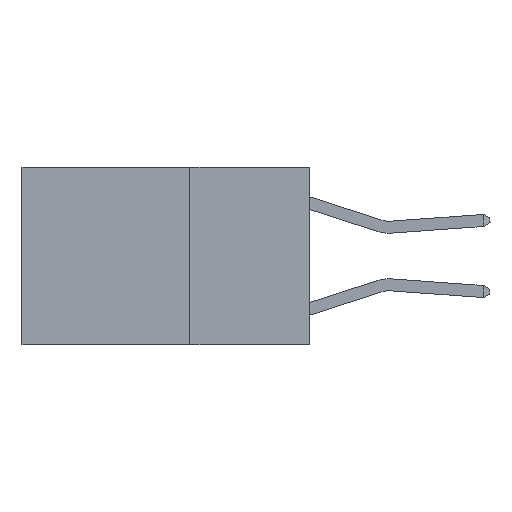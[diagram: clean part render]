
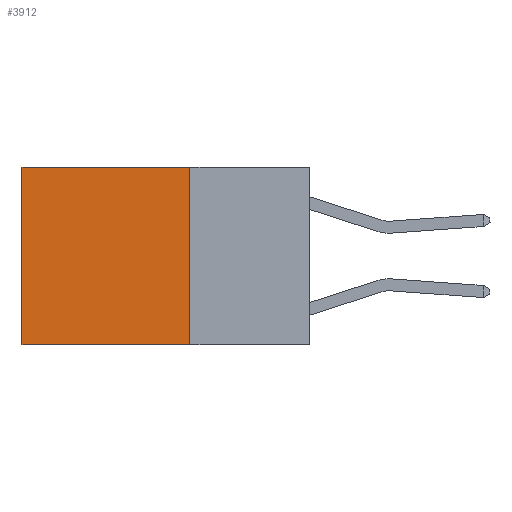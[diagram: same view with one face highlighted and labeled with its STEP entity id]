
A CAD part, left-side view. The second image highlights one B-rep face of the part: STEP entity #3912.
In plain terms, the highlighted planar face has unit normal (-1, 0, 0).
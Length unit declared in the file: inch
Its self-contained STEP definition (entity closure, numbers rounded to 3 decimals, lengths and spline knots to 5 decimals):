
#77 = EDGE_LOOP ( 'NONE', ( #11170, #1168, #11454, #1470 ) ) ;
#141 = VECTOR ( 'NONE', #8031, 39.37008 ) ;
#143 = CARTESIAN_POINT ( 'NONE',  ( 0.2625, 0.6, 0. ) ) ;
#726 = EDGE_CURVE ( 'NONE', #1271, #7814, #10542, .T. ) ;
#819 = EDGE_CURVE ( 'NONE', #9220, #2020, #12403, .T. ) ;
#1168 = ORIENTED_EDGE ( 'NONE', *, *, #726, .F. ) ;
#1271 = VERTEX_POINT ( 'NONE', #5472 ) ;
#1293 = DIRECTION ( 'NONE',  ( 1., 0., 0. ) ) ;
#1423 = FACE_OUTER_BOUND ( 'NONE', #77, .T. ) ;
#1470 = ORIENTED_EDGE ( 'NONE', *, *, #819, .T. ) ;
#2020 = VERTEX_POINT ( 'NONE', #8731 ) ;
#2062 = CARTESIAN_POINT ( 'NONE',  ( 0.2625, 0.25, 0. ) ) ;
#2478 = LINE ( 'NONE', #143, #141 ) ;
#2908 = VECTOR ( 'NONE', #8489, 39.37008 ) ;
#2955 = CARTESIAN_POINT ( 'NONE',  ( 0.2625, 0.25, 0. ) ) ;
#3323 = AXIS2_PLACEMENT_3D ( 'NONE', #2062, #1293, #8204 ) ;
#3598 = CARTESIAN_POINT ( 'NONE',  ( 0.2625, 0.6, -0.37 ) ) ;
#3912 = ADVANCED_FACE ( 'NONE', ( #1423 ), #6130, .F. ) ;
#5231 = VECTOR ( 'NONE', #8505, 39.37008 ) ;
#5472 = CARTESIAN_POINT ( 'NONE',  ( 0.2625, 0.25, -0.37 ) ) ;
#6130 = PLANE ( 'NONE',  #3323 ) ;
#6250 = EDGE_CURVE ( 'NONE', #2020, #7814, #2478, .T. ) ;
#6418 = CARTESIAN_POINT ( 'NONE',  ( 0.2625, 0.25, 0. ) ) ;
#7561 = CARTESIAN_POINT ( 'NONE',  ( 0.2625, 0.25, 0. ) ) ;
#7814 = VERTEX_POINT ( 'NONE', #3598 ) ;
#8031 = DIRECTION ( 'NONE',  ( 0., 0., -1. ) ) ;
#8114 = LINE ( 'NONE', #7561, #2908 ) ;
#8204 = DIRECTION ( 'NONE',  ( 0., 0., -1. ) ) ;
#8330 = VECTOR ( 'NONE', #9864, 39.37008 ) ;
#8489 = DIRECTION ( 'NONE',  ( 0., 0., -1. ) ) ;
#8505 = DIRECTION ( 'NONE',  ( 0., 1., 0. ) ) ;
#8731 = CARTESIAN_POINT ( 'NONE',  ( 0.2625, 0.6, 0. ) ) ;
#9220 = VERTEX_POINT ( 'NONE', #6418 ) ;
#9864 = DIRECTION ( 'NONE',  ( 0., 1., 0. ) ) ;
#10542 = LINE ( 'NONE', #11407, #8330 ) ;
#11170 = ORIENTED_EDGE ( 'NONE', *, *, #6250, .T. ) ;
#11407 = CARTESIAN_POINT ( 'NONE',  ( 0.2625, 0.25, -0.37 ) ) ;
#11454 = ORIENTED_EDGE ( 'NONE', *, *, #12310, .F. ) ;
#12310 = EDGE_CURVE ( 'NONE', #9220, #1271, #8114, .T. ) ;
#12403 = LINE ( 'NONE', #2955, #5231 ) ;
